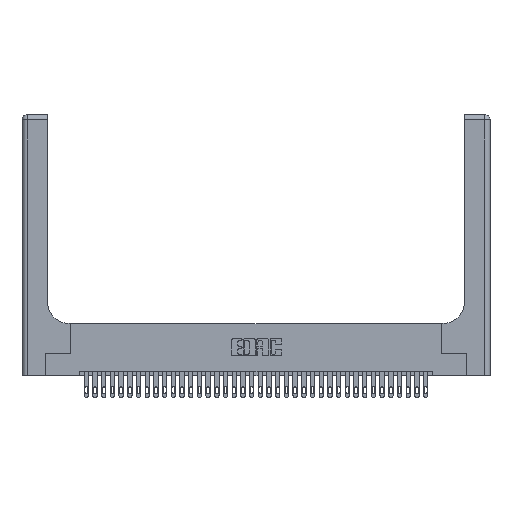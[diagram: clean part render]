
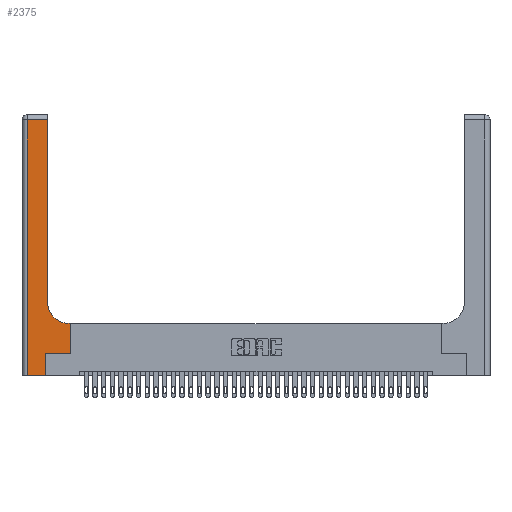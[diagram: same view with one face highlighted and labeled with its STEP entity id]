
A CAD part, top view. The second image highlights one B-rep face of the part: STEP entity #2375.
In plain terms, the highlighted planar face has unit normal (0, 0, 1).
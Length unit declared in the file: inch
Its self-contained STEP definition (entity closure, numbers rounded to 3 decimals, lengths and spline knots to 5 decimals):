
#830 = EDGE_CURVE ( 'NONE', #23036, #34344, #27903, .T. ) ;
#1060 = DIRECTION ( 'NONE',  ( 1., 0., 0. ) ) ;
#2001 = EDGE_CURVE ( 'NONE', #28991, #18294, #9578, .T. ) ;
#2375 = ADVANCED_FACE ( 'NONE', ( #21571 ), #3543, .F. ) ;
#3173 = CARTESIAN_POINT ( 'NONE',  ( 0.5585, 0.6, 0.37 ) ) ;
#3543 = PLANE ( 'NONE',  #31475 ) ;
#4396 = EDGE_CURVE ( 'NONE', #28326, #28991, #7698, .T. ) ;
#4589 = EDGE_CURVE ( 'NONE', #34344, #33453, #29762, .T. ) ;
#5682 = CARTESIAN_POINT ( 'NONE',  ( 0.06, 2.94, 0.37 ) ) ;
#5821 = EDGE_CURVE ( 'NONE', #33453, #24327, #34626, .T. ) ;
#6777 = VECTOR ( 'NONE', #21372, 39.37008 ) ;
#7294 = DIRECTION ( 'NONE',  ( 0., -1., 0. ) ) ;
#7473 = DIRECTION ( 'NONE',  ( -1., 0., 0. ) ) ;
#7514 = ORIENTED_EDGE ( 'NONE', *, *, #4589, .T. ) ;
#7621 = CARTESIAN_POINT ( 'NONE',  ( 0.5585, 0.25, 0.37 ) ) ;
#7698 = LINE ( 'NONE', #26820, #19207 ) ;
#7769 = VERTEX_POINT ( 'NONE', #19677 ) ;
#7943 = LINE ( 'NONE', #29400, #23838 ) ;
#8763 = ORIENTED_EDGE ( 'NONE', *, *, #15464, .T. ) ;
#9166 = CARTESIAN_POINT ( 'NONE',  ( 0.06, 3., 0.37 ) ) ;
#9488 = DIRECTION ( 'NONE',  ( 0., 0., -1. ) ) ;
#9578 = LINE ( 'NONE', #7621, #33142 ) ;
#9580 = AXIS2_PLACEMENT_3D ( 'NONE', #18795, #16073, #19052 ) ;
#10165 = CARTESIAN_POINT ( 'NONE',  ( 0.2915, 0.6, 0.37 ) ) ;
#10274 = CARTESIAN_POINT ( 'NONE',  ( 0.5585, 0.25, 0.37 ) ) ;
#15155 = VECTOR ( 'NONE', #15664, 39.37008 ) ;
#15464 = EDGE_CURVE ( 'NONE', #18294, #23036, #36274, .T. ) ;
#15664 = DIRECTION ( 'NONE',  ( 0., 1., 0. ) ) ;
#15888 = ORIENTED_EDGE ( 'NONE', *, *, #23840, .T. ) ;
#16073 = DIRECTION ( 'NONE',  ( 0., 0., -1. ) ) ;
#16858 = EDGE_CURVE ( 'NONE', #24327, #25641, #25966, .T. ) ;
#17027 = LINE ( 'NONE', #18510, #6777 ) ;
#17343 = CARTESIAN_POINT ( 'NONE',  ( 0., 2.94, 0.37 ) ) ;
#18167 = ORIENTED_EDGE ( 'NONE', *, *, #16858, .T. ) ;
#18294 = VERTEX_POINT ( 'NONE', #3173 ) ;
#18510 = CARTESIAN_POINT ( 'NONE',  ( 0., 0., 0.37 ) ) ;
#18795 = CARTESIAN_POINT ( 'NONE',  ( 0.5415, 0.85, 0.37 ) ) ;
#19018 = CARTESIAN_POINT ( 'NONE',  ( 0.2915, 2.94, 0.37 ) ) ;
#19052 = DIRECTION ( 'NONE',  ( 1., 0., 0. ) ) ;
#19207 = VECTOR ( 'NONE', #1060, 39.37008 ) ;
#19677 = CARTESIAN_POINT ( 'NONE',  ( 0.269, 0., 0.37 ) ) ;
#20190 = DIRECTION ( 'NONE',  ( -1., 0., 0. ) ) ;
#20354 = EDGE_CURVE ( 'NONE', #25641, #7769, #17027, .T. ) ;
#20510 = CARTESIAN_POINT ( 'NONE',  ( 0.2915, 0.85, 0.37 ) ) ;
#21372 = DIRECTION ( 'NONE',  ( 1., 0., 0. ) ) ;
#21571 = FACE_OUTER_BOUND ( 'NONE', #36186, .T. ) ;
#21953 = DIRECTION ( 'NONE',  ( 0., 1., 0. ) ) ;
#22014 = VECTOR ( 'NONE', #7294, 39.37008 ) ;
#23036 = VERTEX_POINT ( 'NONE', #30776 ) ;
#23362 = ORIENTED_EDGE ( 'NONE', *, *, #830, .T. ) ;
#23498 = DIRECTION ( 'NONE',  ( 0., 1., 0. ) ) ;
#23838 = VECTOR ( 'NONE', #23498, 39.37008 ) ;
#23840 = EDGE_CURVE ( 'NONE', #7769, #28326, #7943, .T. ) ;
#24327 = VERTEX_POINT ( 'NONE', #5682 ) ;
#25641 = VERTEX_POINT ( 'NONE', #31505 ) ;
#25966 = LINE ( 'NONE', #9166, #22014 ) ;
#26820 = CARTESIAN_POINT ( 'NONE',  ( 0.269, 0.25, 0.37 ) ) ;
#27057 = VECTOR ( 'NONE', #20190, 39.37008 ) ;
#27618 = DIRECTION ( 'NONE',  ( -1., 0., 0. ) ) ;
#27903 = CIRCLE ( 'NONE', #9580, 0.25 ) ;
#28326 = VERTEX_POINT ( 'NONE', #32049 ) ;
#28342 = ORIENTED_EDGE ( 'NONE', *, *, #20354, .T. ) ;
#28991 = VERTEX_POINT ( 'NONE', #10274 ) ;
#29400 = CARTESIAN_POINT ( 'NONE',  ( 0.269, 0., 0.37 ) ) ;
#29494 = CARTESIAN_POINT ( 'NONE',  ( 0., 3., 0.37 ) ) ;
#29506 = CARTESIAN_POINT ( 'NONE',  ( 0.2915, 3., 0.37 ) ) ;
#29762 = LINE ( 'NONE', #29506, #15155 ) ;
#30776 = CARTESIAN_POINT ( 'NONE',  ( 0.5415, 0.6, 0.37 ) ) ;
#31341 = VECTOR ( 'NONE', #7473, 39.37008 ) ;
#31475 = AXIS2_PLACEMENT_3D ( 'NONE', #29494, #9488, #27618 ) ;
#31505 = CARTESIAN_POINT ( 'NONE',  ( 0.06, 0., 0.37 ) ) ;
#32049 = CARTESIAN_POINT ( 'NONE',  ( 0.269, 0.25, 0.37 ) ) ;
#32553 = ORIENTED_EDGE ( 'NONE', *, *, #5821, .T. ) ;
#33142 = VECTOR ( 'NONE', #21953, 39.37008 ) ;
#33453 = VERTEX_POINT ( 'NONE', #19018 ) ;
#34049 = ORIENTED_EDGE ( 'NONE', *, *, #4396, .T. ) ;
#34344 = VERTEX_POINT ( 'NONE', #20510 ) ;
#34626 = LINE ( 'NONE', #17343, #27057 ) ;
#34907 = ORIENTED_EDGE ( 'NONE', *, *, #2001, .T. ) ;
#36186 = EDGE_LOOP ( 'NONE', ( #7514, #32553, #18167, #28342, #15888, #34049, #34907, #8763, #23362 ) ) ;
#36274 = LINE ( 'NONE', #10165, #31341 ) ;
